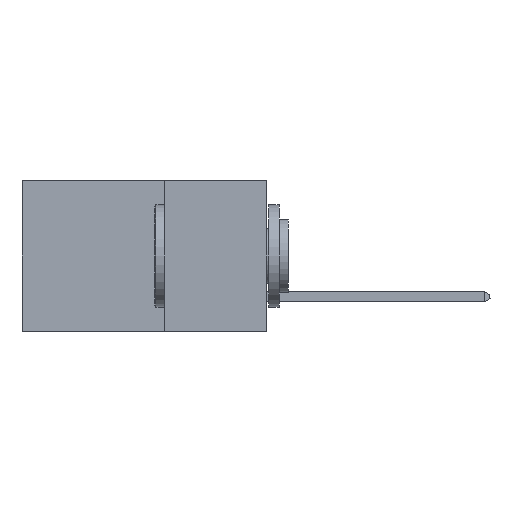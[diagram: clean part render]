
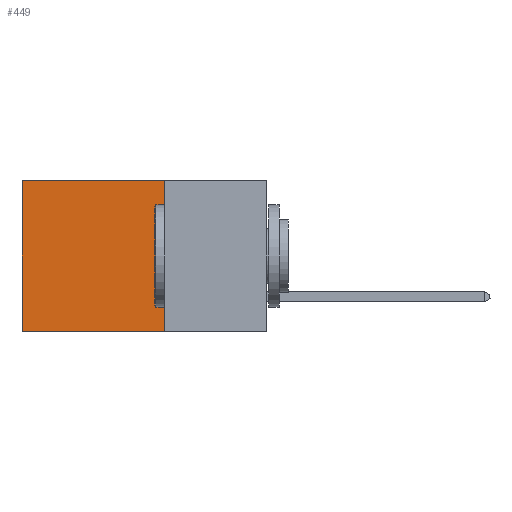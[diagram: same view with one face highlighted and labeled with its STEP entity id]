
A CAD part, left-side view. The second image highlights one B-rep face of the part: STEP entity #449.
In plain terms, the highlighted planar face has unit normal (-1, 0, 0).
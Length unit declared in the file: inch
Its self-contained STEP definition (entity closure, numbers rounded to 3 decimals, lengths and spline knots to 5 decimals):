
#449 = ADVANCED_FACE ( 'NONE', ( #13526 ), #25091, .F. ) ;
#1620 = VECTOR ( 'NONE', #22835, 39.37008 ) ;
#1906 = EDGE_CURVE ( 'NONE', #29014, #39405, #40612, .T. ) ;
#2112 = LINE ( 'NONE', #22971, #1620 ) ;
#3418 = DIRECTION ( 'NONE',  ( 0., 1., 0. ) ) ;
#4943 = DIRECTION ( 'NONE',  ( 0., 0., -1. ) ) ;
#5092 = DIRECTION ( 'NONE',  ( 1., 0., 0. ) ) ;
#5994 = VERTEX_POINT ( 'NONE', #34710 ) ;
#7097 = EDGE_CURVE ( 'NONE', #33636, #39405, #2112, .T. ) ;
#7497 = ORIENTED_EDGE ( 'NONE', *, *, #24844, .T. ) ;
#8109 = CARTESIAN_POINT ( 'NONE',  ( 0.2875, 0.6, 0. ) ) ;
#8595 = CARTESIAN_POINT ( 'NONE',  ( 0.2875, 0.25, 0. ) ) ;
#10407 = DIRECTION ( 'NONE',  ( 0., 1., 0. ) ) ;
#11892 = VECTOR ( 'NONE', #10407, 39.37008 ) ;
#12811 = ORIENTED_EDGE ( 'NONE', *, *, #1906, .F. ) ;
#13091 = CARTESIAN_POINT ( 'NONE',  ( 0.2875, 0.25, 0. ) ) ;
#13526 = FACE_OUTER_BOUND ( 'NONE', #16631, .T. ) ;
#16631 = EDGE_LOOP ( 'NONE', ( #35151, #12811, #35493, #7497 ) ) ;
#19653 = EDGE_CURVE ( 'NONE', #5994, #29014, #40159, .T. ) ;
#20242 = CARTESIAN_POINT ( 'NONE',  ( 0.2875, 0.25, -0.37 ) ) ;
#20290 = CARTESIAN_POINT ( 'NONE',  ( 0.2875, 0.6, -0.37 ) ) ;
#22835 = DIRECTION ( 'NONE',  ( 0., 0., -1. ) ) ;
#22971 = CARTESIAN_POINT ( 'NONE',  ( 0.2875, 0.6, 0. ) ) ;
#23451 = LINE ( 'NONE', #13091, #11892 ) ;
#23688 = CARTESIAN_POINT ( 'NONE',  ( 0.2875, 0.25, -0.37 ) ) ;
#24655 = CARTESIAN_POINT ( 'NONE',  ( 0.2875, 0.25, 0. ) ) ;
#24844 = EDGE_CURVE ( 'NONE', #5994, #33636, #23451, .T. ) ;
#25091 = PLANE ( 'NONE',  #39186 ) ;
#28721 = DIRECTION ( 'NONE',  ( 0., 0., -1. ) ) ;
#29014 = VERTEX_POINT ( 'NONE', #20242 ) ;
#30185 = VECTOR ( 'NONE', #3418, 39.37008 ) ;
#31272 = VECTOR ( 'NONE', #28721, 39.37008 ) ;
#33636 = VERTEX_POINT ( 'NONE', #8109 ) ;
#34710 = CARTESIAN_POINT ( 'NONE',  ( 0.2875, 0.25, 0. ) ) ;
#35151 = ORIENTED_EDGE ( 'NONE', *, *, #7097, .T. ) ;
#35493 = ORIENTED_EDGE ( 'NONE', *, *, #19653, .F. ) ;
#39186 = AXIS2_PLACEMENT_3D ( 'NONE', #24655, #5092, #4943 ) ;
#39405 = VERTEX_POINT ( 'NONE', #20290 ) ;
#40159 = LINE ( 'NONE', #8595, #31272 ) ;
#40612 = LINE ( 'NONE', #23688, #30185 ) ;
